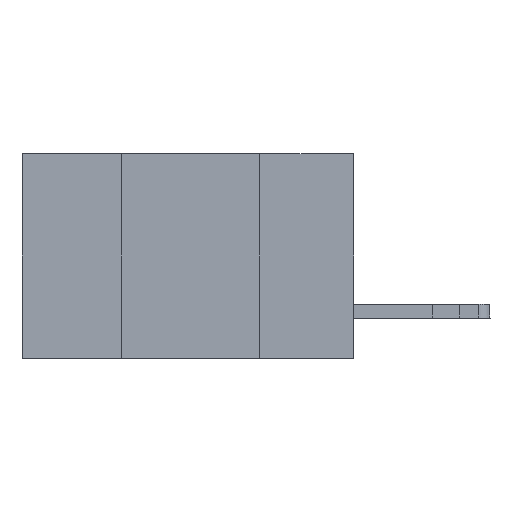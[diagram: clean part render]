
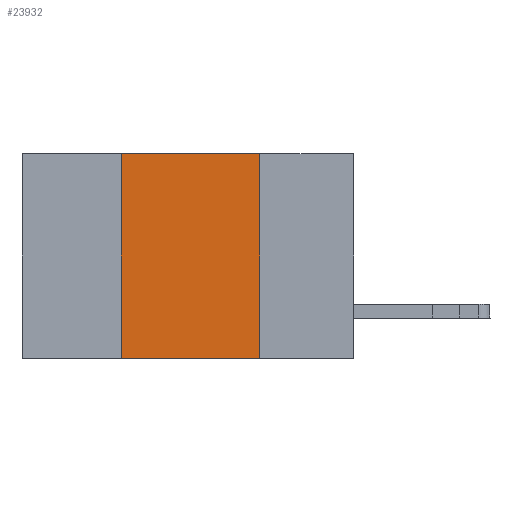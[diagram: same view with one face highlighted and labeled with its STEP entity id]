
A CAD part, left-side view. The second image highlights one B-rep face of the part: STEP entity #23932.
In plain terms, the highlighted planar face has unit normal (-1, 0, 0).
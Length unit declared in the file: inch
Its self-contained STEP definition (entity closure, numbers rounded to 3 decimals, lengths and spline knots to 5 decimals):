
#875 = CARTESIAN_POINT ( 'NONE',  ( 0., 0.6, -0.37 ) ) ;
#1456 = VERTEX_POINT ( 'NONE', #9183 ) ;
#1962 = CARTESIAN_POINT ( 'NONE',  ( 0., 0.6, 0. ) ) ;
#2598 = VECTOR ( 'NONE', #17866, 39.37008 ) ;
#2714 = CARTESIAN_POINT ( 'NONE',  ( 0., 0.17, 0. ) ) ;
#2969 = CARTESIAN_POINT ( 'NONE',  ( 0., 0.42, 0. ) ) ;
#5899 = VECTOR ( 'NONE', #23510, 39.37008 ) ;
#6646 = CARTESIAN_POINT ( 'NONE',  ( 0., 0.42, -0.37 ) ) ;
#6925 = FACE_OUTER_BOUND ( 'NONE', #19411, .T. ) ;
#8907 = LINE ( 'NONE', #875, #2598 ) ;
#9121 = DIRECTION ( 'NONE',  ( 0., 0., -1. ) ) ;
#9183 = CARTESIAN_POINT ( 'NONE',  ( 0., 0.17, 0. ) ) ;
#10539 = PLANE ( 'NONE',  #16712 ) ;
#11228 = VERTEX_POINT ( 'NONE', #23280 ) ;
#11601 = LINE ( 'NONE', #21408, #5899 ) ;
#12676 = DIRECTION ( 'NONE',  ( 0., 0., -1. ) ) ;
#13378 = VERTEX_POINT ( 'NONE', #6646 ) ;
#13389 = EDGE_CURVE ( 'NONE', #13378, #26928, #11601, .T. ) ;
#13704 = ORIENTED_EDGE ( 'NONE', *, *, #13389, .F. ) ;
#14326 = DIRECTION ( 'NONE',  ( 0., -1., 0. ) ) ;
#16323 = EDGE_CURVE ( 'NONE', #26928, #1456, #22852, .T. ) ;
#16712 = AXIS2_PLACEMENT_3D ( 'NONE', #1962, #25198, #12676 ) ;
#17866 = DIRECTION ( 'NONE',  ( 0., -1., 0. ) ) ;
#18629 = EDGE_CURVE ( 'NONE', #13378, #11228, #8907, .T. ) ;
#18946 = ORIENTED_EDGE ( 'NONE', *, *, #20984, .F. ) ;
#19397 = LINE ( 'NONE', #2714, #23608 ) ;
#19411 = EDGE_LOOP ( 'NONE', ( #18946, #20055, #13704, #22477 ) ) ;
#20055 = ORIENTED_EDGE ( 'NONE', *, *, #16323, .F. ) ;
#20984 = EDGE_CURVE ( 'NONE', #1456, #11228, #19397, .T. ) ;
#21408 = CARTESIAN_POINT ( 'NONE',  ( 0., 0.42, 0. ) ) ;
#22477 = ORIENTED_EDGE ( 'NONE', *, *, #18629, .T. ) ;
#22852 = LINE ( 'NONE', #26824, #23511 ) ;
#23280 = CARTESIAN_POINT ( 'NONE',  ( 0., 0.17, -0.37 ) ) ;
#23510 = DIRECTION ( 'NONE',  ( 0., 0., 1. ) ) ;
#23511 = VECTOR ( 'NONE', #14326, 39.37008 ) ;
#23608 = VECTOR ( 'NONE', #9121, 39.37008 ) ;
#23932 = ADVANCED_FACE ( 'NONE', ( #6925 ), #10539, .F. ) ;
#25198 = DIRECTION ( 'NONE',  ( 1., 0., 0. ) ) ;
#26824 = CARTESIAN_POINT ( 'NONE',  ( 0., 0.6, 0. ) ) ;
#26928 = VERTEX_POINT ( 'NONE', #2969 ) ;
